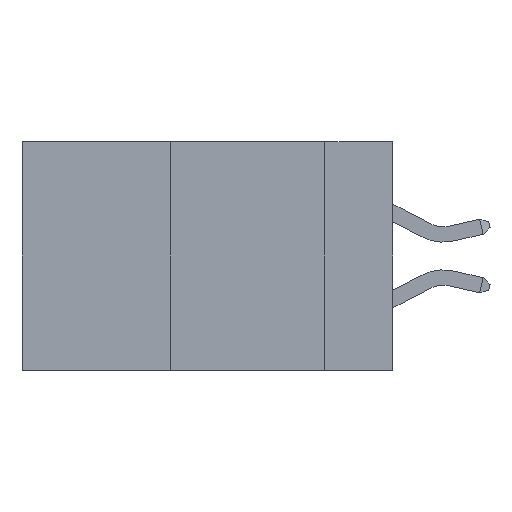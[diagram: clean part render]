
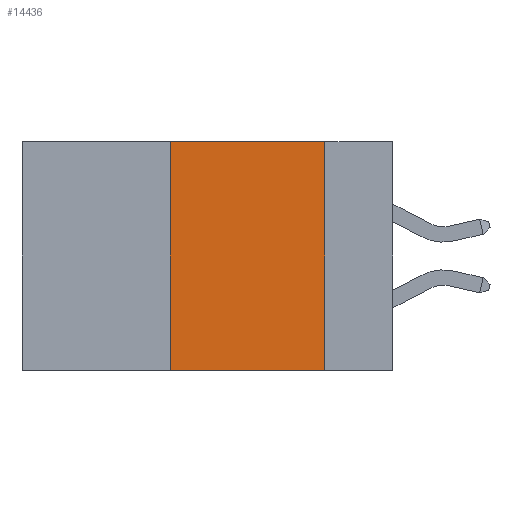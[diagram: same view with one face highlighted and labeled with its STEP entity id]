
A CAD part, left-side view. The second image highlights one B-rep face of the part: STEP entity #14436.
In plain terms, the highlighted planar face has unit normal (-1, 0, 0).
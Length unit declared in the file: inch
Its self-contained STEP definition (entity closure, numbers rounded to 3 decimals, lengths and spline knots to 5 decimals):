
#464 = CARTESIAN_POINT ( 'NONE',  ( 0., 0.6, 0. ) ) ;
#524 = CARTESIAN_POINT ( 'NONE',  ( 0., 0.36, 0. ) ) ;
#530 = VERTEX_POINT ( 'NONE', #1826 ) ;
#1206 = DIRECTION ( 'NONE',  ( 1., 0., 0. ) ) ;
#1208 = ORIENTED_EDGE ( 'NONE', *, *, #5473, .F. ) ;
#1456 = EDGE_CURVE ( 'NONE', #5834, #9916, #12004, .T. ) ;
#1555 = CARTESIAN_POINT ( 'NONE',  ( 0., 0.6, -0.37 ) ) ;
#1751 = CARTESIAN_POINT ( 'NONE',  ( 0., 0.36, -0.37 ) ) ;
#1826 = CARTESIAN_POINT ( 'NONE',  ( 0., 0.36, 0. ) ) ;
#2391 = DIRECTION ( 'NONE',  ( 0., 0., -1. ) ) ;
#3077 = ORIENTED_EDGE ( 'NONE', *, *, #10624, .F. ) ;
#3085 = VECTOR ( 'NONE', #13933, 39.37008 ) ;
#3519 = FACE_OUTER_BOUND ( 'NONE', #11135, .T. ) ;
#3842 = CARTESIAN_POINT ( 'NONE',  ( 0., 0.11, -0.37 ) ) ;
#4079 = DIRECTION ( 'NONE',  ( 0., -1., 0. ) ) ;
#4420 = EDGE_CURVE ( 'NONE', #6812, #9916, #7916, .T. ) ;
#4984 = VECTOR ( 'NONE', #4079, 39.37008 ) ;
#5473 = EDGE_CURVE ( 'NONE', #5834, #530, #7889, .T. ) ;
#5573 = AXIS2_PLACEMENT_3D ( 'NONE', #7475, #1206, #10081 ) ;
#5834 = VERTEX_POINT ( 'NONE', #1751 ) ;
#6207 = PLANE ( 'NONE',  #5573 ) ;
#6812 = VERTEX_POINT ( 'NONE', #9143 ) ;
#7475 = CARTESIAN_POINT ( 'NONE',  ( 0., 0.6, 0. ) ) ;
#7889 = LINE ( 'NONE', #524, #13849 ) ;
#7916 = LINE ( 'NONE', #15007, #9919 ) ;
#8427 = ORIENTED_EDGE ( 'NONE', *, *, #1456, .T. ) ;
#9143 = CARTESIAN_POINT ( 'NONE',  ( 0., 0.11, 0. ) ) ;
#9567 = DIRECTION ( 'NONE',  ( 0., 0., 1. ) ) ;
#9916 = VERTEX_POINT ( 'NONE', #3842 ) ;
#9919 = VECTOR ( 'NONE', #2391, 39.37008 ) ;
#10081 = DIRECTION ( 'NONE',  ( 0., 0., -1. ) ) ;
#10624 = EDGE_CURVE ( 'NONE', #530, #6812, #13489, .T. ) ;
#11135 = EDGE_LOOP ( 'NONE', ( #11543, #3077, #1208, #8427 ) ) ;
#11543 = ORIENTED_EDGE ( 'NONE', *, *, #4420, .F. ) ;
#12004 = LINE ( 'NONE', #1555, #3085 ) ;
#13489 = LINE ( 'NONE', #464, #4984 ) ;
#13849 = VECTOR ( 'NONE', #9567, 39.37008 ) ;
#13933 = DIRECTION ( 'NONE',  ( 0., -1., 0. ) ) ;
#14436 = ADVANCED_FACE ( 'NONE', ( #3519 ), #6207, .F. ) ;
#15007 = CARTESIAN_POINT ( 'NONE',  ( 0., 0.11, 0. ) ) ;
